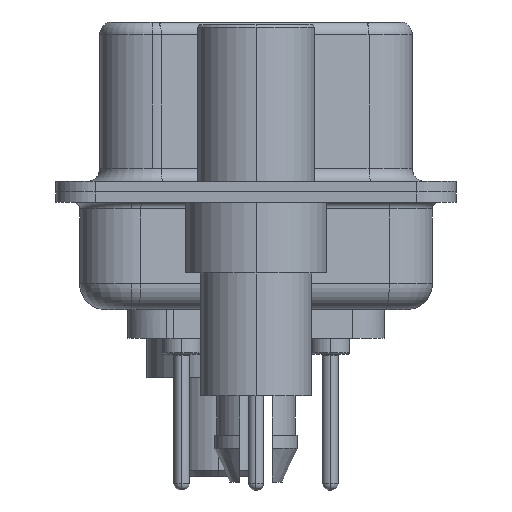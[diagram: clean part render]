
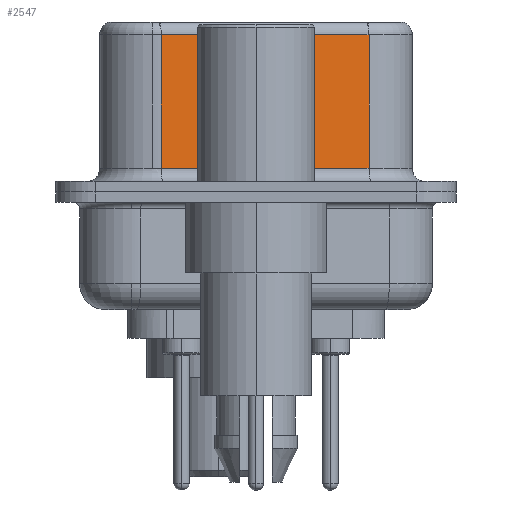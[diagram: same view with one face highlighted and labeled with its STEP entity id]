
A CAD part, left-side view. The second image highlights one B-rep face of the part: STEP entity #2547.
In plain terms, the highlighted planar face has unit normal (-0.985, -0.174, 0).
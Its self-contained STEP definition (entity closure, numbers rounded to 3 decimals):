
#653 = CARTESIAN_POINT ( 'NONE',  ( 5.132, -4.322, 0.9 ) ) ;
#728 = DIRECTION ( 'NONE',  ( 0., 0., -1. ) ) ;
#1281 = CARTESIAN_POINT ( 'NONE',  ( 5.132, -4.322, 6.02 ) ) ;
#1965 = EDGE_CURVE ( 'NONE', #22956, #21787, #28668, .T. ) ;
#2547 = ADVANCED_FACE ( 'NONE', ( #27935 ), #26698, .F. ) ;
#4190 = EDGE_CURVE ( 'NONE', #21787, #19239, #27863, .T. ) ;
#4413 = CARTESIAN_POINT ( 'NONE',  ( 3.73, 3.628, 6.02 ) ) ;
#5277 = CARTESIAN_POINT ( 'NONE',  ( 5.132, -4.322, 0.9 ) ) ;
#9240 = VERTEX_POINT ( 'NONE', #653 ) ;
#9827 = AXIS2_PLACEMENT_3D ( 'NONE', #14263, #26405, #26274 ) ;
#10466 = LINE ( 'NONE', #5277, #22149 ) ;
#11781 = VECTOR ( 'NONE', #22394, 1000. ) ;
#13595 = ORIENTED_EDGE ( 'NONE', *, *, #15925, .T. ) ;
#14177 = CARTESIAN_POINT ( 'NONE',  ( 5.132, -4.322, 6.52 ) ) ;
#14263 = CARTESIAN_POINT ( 'NONE',  ( 5.132, -4.322, 6.52 ) ) ;
#15925 = EDGE_CURVE ( 'NONE', #19239, #9240, #10466, .T. ) ;
#17038 = VECTOR ( 'NONE', #23474, 1000. ) ;
#18519 = DIRECTION ( 'NONE',  ( 0.174, -0.985, 0. ) ) ;
#18711 = ORIENTED_EDGE ( 'NONE', *, *, #4190, .T. ) ;
#19239 = VERTEX_POINT ( 'NONE', #27233 ) ;
#19291 = ORIENTED_EDGE ( 'NONE', *, *, #20316, .F. ) ;
#20316 = EDGE_CURVE ( 'NONE', #22956, #9240, #27721, .T. ) ;
#20513 = EDGE_LOOP ( 'NONE', ( #19291, #20767, #18711, #13595 ) ) ;
#20767 = ORIENTED_EDGE ( 'NONE', *, *, #1965, .T. ) ;
#21787 = VERTEX_POINT ( 'NONE', #4413 ) ;
#22149 = VECTOR ( 'NONE', #18519, 1000. ) ;
#22394 = DIRECTION ( 'NONE',  ( 0., 0., -1. ) ) ;
#22956 = VERTEX_POINT ( 'NONE', #23591 ) ;
#23474 = DIRECTION ( 'NONE',  ( -0.174, 0.985, 0. ) ) ;
#23591 = CARTESIAN_POINT ( 'NONE',  ( 5.132, -4.322, 6.02 ) ) ;
#24555 = CARTESIAN_POINT ( 'NONE',  ( 3.73, 3.628, 6.52 ) ) ;
#26274 = DIRECTION ( 'NONE',  ( -0.174, 0.985, 0. ) ) ;
#26405 = DIRECTION ( 'NONE',  ( 0.985, 0.174, 0. ) ) ;
#26698 = PLANE ( 'NONE',  #9827 ) ;
#27233 = CARTESIAN_POINT ( 'NONE',  ( 3.73, 3.628, 0.9 ) ) ;
#27721 = LINE ( 'NONE', #14177, #28422 ) ;
#27863 = LINE ( 'NONE', #24555, #11781 ) ;
#27935 = FACE_OUTER_BOUND ( 'NONE', #20513, .T. ) ;
#28422 = VECTOR ( 'NONE', #728, 1000. ) ;
#28668 = LINE ( 'NONE', #1281, #17038 ) ;
